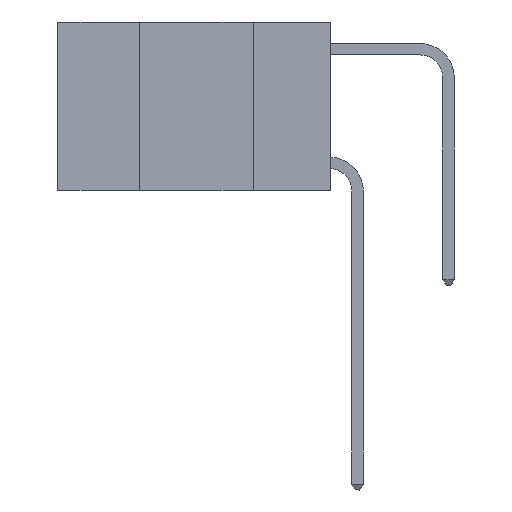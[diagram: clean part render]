
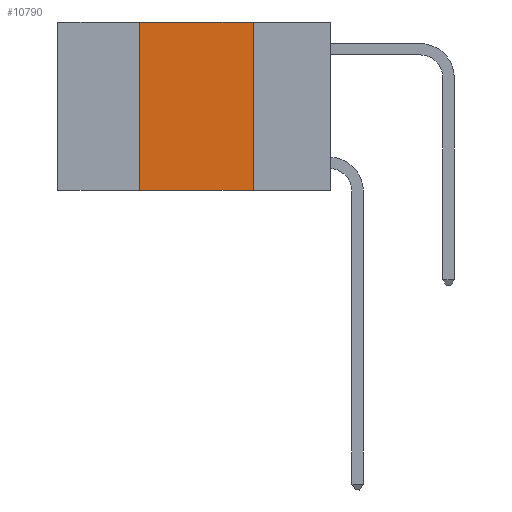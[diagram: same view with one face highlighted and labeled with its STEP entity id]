
A CAD part, left-side view. The second image highlights one B-rep face of the part: STEP entity #10790.
In plain terms, the highlighted planar face has unit normal (-1, 0, 0).
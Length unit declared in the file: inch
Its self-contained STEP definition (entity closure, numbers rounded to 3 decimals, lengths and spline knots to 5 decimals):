
#443 = VECTOR ( 'NONE', #21036, 39.37008 ) ;
#912 = EDGE_CURVE ( 'NONE', #15316, #17242, #10173, .T. ) ;
#1840 = DIRECTION ( 'NONE',  ( 0., -1., 0. ) ) ;
#2418 = FACE_OUTER_BOUND ( 'NONE', #13761, .T. ) ;
#2862 = ORIENTED_EDGE ( 'NONE', *, *, #912, .F. ) ;
#4173 = CARTESIAN_POINT ( 'NONE',  ( 0., 0.6, 0. ) ) ;
#4562 = LINE ( 'NONE', #13113, #12585 ) ;
#5105 = CARTESIAN_POINT ( 'NONE',  ( 0., 0.42, 0. ) ) ;
#5261 = CARTESIAN_POINT ( 'NONE',  ( 0., 0.17, 0. ) ) ;
#5605 = VECTOR ( 'NONE', #1840, 39.37008 ) ;
#6629 = VECTOR ( 'NONE', #8789, 39.37008 ) ;
#8055 = ORIENTED_EDGE ( 'NONE', *, *, #20614, .F. ) ;
#8666 = CARTESIAN_POINT ( 'NONE',  ( 0., 0.42, -0.37 ) ) ;
#8789 = DIRECTION ( 'NONE',  ( 0., -1., 0. ) ) ;
#9920 = DIRECTION ( 'NONE',  ( 1., 0., 0. ) ) ;
#10173 = LINE ( 'NONE', #4173, #5605 ) ;
#10790 = ADVANCED_FACE ( 'NONE', ( #2418 ), #19991, .F. ) ;
#12585 = VECTOR ( 'NONE', #14896, 39.37008 ) ;
#12686 = ORIENTED_EDGE ( 'NONE', *, *, #18387, .F. ) ;
#13113 = CARTESIAN_POINT ( 'NONE',  ( 0., 0.17, 0. ) ) ;
#13761 = EDGE_LOOP ( 'NONE', ( #8055, #2862, #12686, #16566 ) ) ;
#14784 = LINE ( 'NONE', #19363, #443 ) ;
#14896 = DIRECTION ( 'NONE',  ( 0., 0., -1. ) ) ;
#15316 = VERTEX_POINT ( 'NONE', #5105 ) ;
#15697 = LINE ( 'NONE', #17245, #6629 ) ;
#16566 = ORIENTED_EDGE ( 'NONE', *, *, #17272, .T. ) ;
#16664 = CARTESIAN_POINT ( 'NONE',  ( 0., 0.6, 0. ) ) ;
#17242 = VERTEX_POINT ( 'NONE', #5261 ) ;
#17245 = CARTESIAN_POINT ( 'NONE',  ( 0., 0.6, -0.37 ) ) ;
#17272 = EDGE_CURVE ( 'NONE', #20268, #20195, #15697, .T. ) ;
#18387 = EDGE_CURVE ( 'NONE', #20268, #15316, #14784, .T. ) ;
#19363 = CARTESIAN_POINT ( 'NONE',  ( 0., 0.42, 0. ) ) ;
#19991 = PLANE ( 'NONE',  #20568 ) ;
#20195 = VERTEX_POINT ( 'NONE', #21888 ) ;
#20268 = VERTEX_POINT ( 'NONE', #8666 ) ;
#20568 = AXIS2_PLACEMENT_3D ( 'NONE', #16664, #9920, #21658 ) ;
#20614 = EDGE_CURVE ( 'NONE', #17242, #20195, #4562, .T. ) ;
#21036 = DIRECTION ( 'NONE',  ( 0., 0., 1. ) ) ;
#21658 = DIRECTION ( 'NONE',  ( 0., 0., -1. ) ) ;
#21888 = CARTESIAN_POINT ( 'NONE',  ( 0., 0.17, -0.37 ) ) ;
